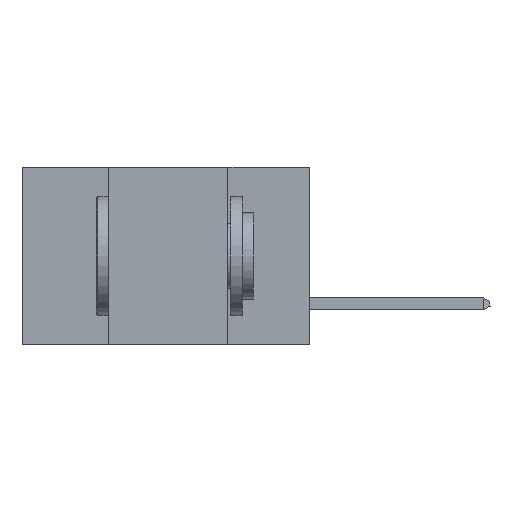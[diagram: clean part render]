
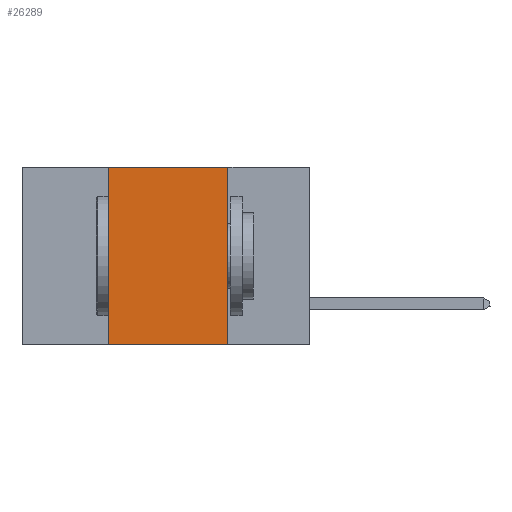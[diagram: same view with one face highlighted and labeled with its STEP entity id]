
A CAD part, left-side view. The second image highlights one B-rep face of the part: STEP entity #26289.
In plain terms, the highlighted planar face has unit normal (-1, 0, 0).
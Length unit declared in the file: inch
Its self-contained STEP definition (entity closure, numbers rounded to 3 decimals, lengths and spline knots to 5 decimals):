
#1752 = PLANE ( 'NONE',  #24055 ) ;
#1841 = EDGE_CURVE ( 'NONE', #9580, #9564, #23016, .T. ) ;
#6327 = EDGE_LOOP ( 'NONE', ( #18646, #22345, #17569, #25358 ) ) ;
#7135 = VECTOR ( 'NONE', #12477, 39.37008 ) ;
#8048 = DIRECTION ( 'NONE',  ( 0., -1., 0. ) ) ;
#8300 = VECTOR ( 'NONE', #28451, 39.37008 ) ;
#8889 = DIRECTION ( 'NONE',  ( 0., 0., -1. ) ) ;
#8926 = CARTESIAN_POINT ( 'NONE',  ( 0., 0.42, -0.37 ) ) ;
#9183 = DIRECTION ( 'NONE',  ( 1., 0., 0. ) ) ;
#9564 = VERTEX_POINT ( 'NONE', #25596 ) ;
#9580 = VERTEX_POINT ( 'NONE', #25695 ) ;
#10881 = FACE_OUTER_BOUND ( 'NONE', #6327, .T. ) ;
#11827 = CARTESIAN_POINT ( 'NONE',  ( 0., 0.6, -0.37 ) ) ;
#12477 = DIRECTION ( 'NONE',  ( 0., 0., 1. ) ) ;
#13830 = CARTESIAN_POINT ( 'NONE',  ( 0., 0.6, 0. ) ) ;
#13914 = LINE ( 'NONE', #11827, #8300 ) ;
#17485 = VECTOR ( 'NONE', #8048, 39.37008 ) ;
#17569 = ORIENTED_EDGE ( 'NONE', *, *, #25178, .F. ) ;
#18437 = VECTOR ( 'NONE', #8889, 39.37008 ) ;
#18646 = ORIENTED_EDGE ( 'NONE', *, *, #27959, .F. ) ;
#22345 = ORIENTED_EDGE ( 'NONE', *, *, #1841, .F. ) ;
#23016 = LINE ( 'NONE', #13830, #17485 ) ;
#23139 = CARTESIAN_POINT ( 'NONE',  ( 0., 0.17, 0. ) ) ;
#23441 = CARTESIAN_POINT ( 'NONE',  ( 0., 0.6, 0. ) ) ;
#24055 = AXIS2_PLACEMENT_3D ( 'NONE', #23441, #9183, #25845 ) ;
#24719 = CARTESIAN_POINT ( 'NONE',  ( 0., 0.17, -0.37 ) ) ;
#25178 = EDGE_CURVE ( 'NONE', #29697, #9580, #26194, .T. ) ;
#25358 = ORIENTED_EDGE ( 'NONE', *, *, #28548, .T. ) ;
#25596 = CARTESIAN_POINT ( 'NONE',  ( 0., 0.17, 0. ) ) ;
#25695 = CARTESIAN_POINT ( 'NONE',  ( 0., 0.42, 0. ) ) ;
#25845 = DIRECTION ( 'NONE',  ( 0., 0., -1. ) ) ;
#26002 = VERTEX_POINT ( 'NONE', #24719 ) ;
#26194 = LINE ( 'NONE', #26710, #7135 ) ;
#26289 = ADVANCED_FACE ( 'NONE', ( #10881 ), #1752, .F. ) ;
#26710 = CARTESIAN_POINT ( 'NONE',  ( 0., 0.42, 0. ) ) ;
#27959 = EDGE_CURVE ( 'NONE', #9564, #26002, #31042, .T. ) ;
#28451 = DIRECTION ( 'NONE',  ( 0., -1., 0. ) ) ;
#28548 = EDGE_CURVE ( 'NONE', #29697, #26002, #13914, .T. ) ;
#29697 = VERTEX_POINT ( 'NONE', #8926 ) ;
#31042 = LINE ( 'NONE', #23139, #18437 ) ;
